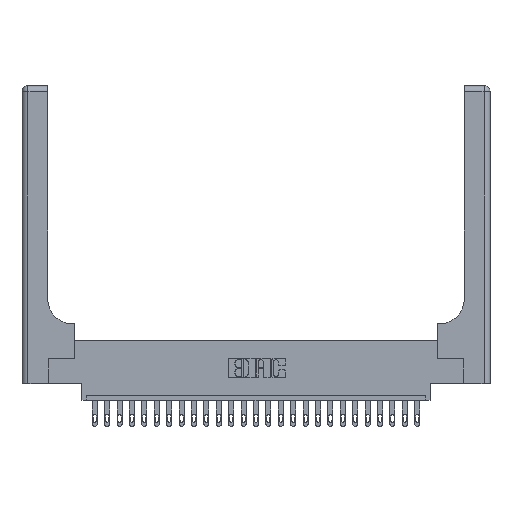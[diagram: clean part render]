
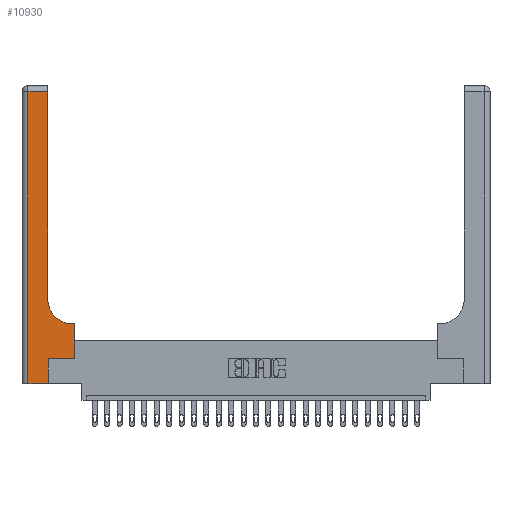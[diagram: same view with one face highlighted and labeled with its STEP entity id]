
A CAD part, top view. The second image highlights one B-rep face of the part: STEP entity #10930.
In plain terms, the highlighted planar face has unit normal (0, 0, 1).
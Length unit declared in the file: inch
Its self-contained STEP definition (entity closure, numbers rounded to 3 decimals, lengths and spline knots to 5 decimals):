
#193 = DIRECTION ( 'NONE',  ( 0., -1., 0. ) ) ;
#1025 = VECTOR ( 'NONE', #5965, 39.37008 ) ;
#1314 = CARTESIAN_POINT ( 'NONE',  ( 0.26, 3., 0.37 ) ) ;
#2083 = VERTEX_POINT ( 'NONE', #12073 ) ;
#2112 = CARTESIAN_POINT ( 'NONE',  ( 0.26, 0.6, 0.37 ) ) ;
#2118 = CARTESIAN_POINT ( 'NONE',  ( 0., 0., 0.37 ) ) ;
#2590 = ORIENTED_EDGE ( 'NONE', *, *, #4494, .T. ) ;
#2878 = CIRCLE ( 'NONE', #19858, 0.25 ) ;
#3769 = DIRECTION ( 'NONE',  ( 0., 0., -1. ) ) ;
#4019 = VERTEX_POINT ( 'NONE', #12612 ) ;
#4285 = CARTESIAN_POINT ( 'NONE',  ( 0.06, 3., 0.37 ) ) ;
#4494 = EDGE_CURVE ( 'NONE', #22353, #8426, #23969, .T. ) ;
#4705 = VERTEX_POINT ( 'NONE', #7761 ) ;
#5190 = LINE ( 'NONE', #10994, #24122 ) ;
#5436 = ORIENTED_EDGE ( 'NONE', *, *, #13300, .T. ) ;
#5561 = EDGE_CURVE ( 'NONE', #14327, #8097, #8085, .T. ) ;
#5607 = CARTESIAN_POINT ( 'NONE',  ( 0.265, 0.25, 0.37 ) ) ;
#5965 = DIRECTION ( 'NONE',  ( 1., 0., 0. ) ) ;
#6201 = CARTESIAN_POINT ( 'NONE',  ( 0.265, 0.25, 0.37 ) ) ;
#7761 = CARTESIAN_POINT ( 'NONE',  ( 0.528, 0.6, 0.37 ) ) ;
#8085 = LINE ( 'NONE', #2118, #1025 ) ;
#8097 = VERTEX_POINT ( 'NONE', #18215 ) ;
#8426 = VERTEX_POINT ( 'NONE', #12751 ) ;
#8872 = ORIENTED_EDGE ( 'NONE', *, *, #14908, .T. ) ;
#9012 = AXIS2_PLACEMENT_3D ( 'NONE', #9348, #3769, #18844 ) ;
#9214 = VECTOR ( 'NONE', #193, 39.37008 ) ;
#9348 = CARTESIAN_POINT ( 'NONE',  ( 0., 3., 0.37 ) ) ;
#10297 = CARTESIAN_POINT ( 'NONE',  ( 0.26, 2.94, 0.37 ) ) ;
#10626 = DIRECTION ( 'NONE',  ( 0., 1., 0. ) ) ;
#10748 = LINE ( 'NONE', #16184, #13868 ) ;
#10930 = ADVANCED_FACE ( 'NONE', ( #11815 ), #19348, .F. ) ;
#10994 = CARTESIAN_POINT ( 'NONE',  ( 0.528, 0.25, 0.37 ) ) ;
#11377 = ORIENTED_EDGE ( 'NONE', *, *, #5561, .T. ) ;
#11395 = DIRECTION ( 'NONE',  ( -1., 0., 0. ) ) ;
#11425 = VECTOR ( 'NONE', #15030, 39.37008 ) ;
#11815 = FACE_OUTER_BOUND ( 'NONE', #22078, .T. ) ;
#12008 = EDGE_CURVE ( 'NONE', #17286, #22353, #12692, .T. ) ;
#12073 = CARTESIAN_POINT ( 'NONE',  ( 0.528, 0.25, 0.37 ) ) ;
#12216 = CARTESIAN_POINT ( 'NONE',  ( 0.51, 0.85, 0.37 ) ) ;
#12612 = CARTESIAN_POINT ( 'NONE',  ( 0.51, 0.6, 0.37 ) ) ;
#12692 = LINE ( 'NONE', #1314, #11425 ) ;
#12751 = CARTESIAN_POINT ( 'NONE',  ( 0.06, 2.94, 0.37 ) ) ;
#13104 = VERTEX_POINT ( 'NONE', #6201 ) ;
#13300 = EDGE_CURVE ( 'NONE', #2083, #4705, #5190, .T. ) ;
#13559 = VECTOR ( 'NONE', #22098, 39.37008 ) ;
#13868 = VECTOR ( 'NONE', #10626, 39.37008 ) ;
#14327 = VERTEX_POINT ( 'NONE', #21493 ) ;
#14553 = CARTESIAN_POINT ( 'NONE',  ( 0., 2.94, 0.37 ) ) ;
#14908 = EDGE_CURVE ( 'NONE', #13104, #2083, #23933, .T. ) ;
#15030 = DIRECTION ( 'NONE',  ( 0., 1., 0. ) ) ;
#15076 = VECTOR ( 'NONE', #22183, 39.37008 ) ;
#15535 = VECTOR ( 'NONE', #11395, 39.37008 ) ;
#15697 = DIRECTION ( 'NONE',  ( 0., 0., -1. ) ) ;
#15782 = LINE ( 'NONE', #4285, #9214 ) ;
#15858 = EDGE_CURVE ( 'NONE', #8426, #14327, #15782, .T. ) ;
#15927 = ORIENTED_EDGE ( 'NONE', *, *, #15858, .T. ) ;
#15940 = CARTESIAN_POINT ( 'NONE',  ( 0.26, 0.85, 0.37 ) ) ;
#16184 = CARTESIAN_POINT ( 'NONE',  ( 0.265, 0., 0.37 ) ) ;
#17286 = VERTEX_POINT ( 'NONE', #15940 ) ;
#17294 = EDGE_CURVE ( 'NONE', #4019, #17286, #2878, .T. ) ;
#17616 = ORIENTED_EDGE ( 'NONE', *, *, #17294, .T. ) ;
#17698 = ORIENTED_EDGE ( 'NONE', *, *, #12008, .T. ) ;
#18037 = ORIENTED_EDGE ( 'NONE', *, *, #22919, .T. ) ;
#18067 = EDGE_CURVE ( 'NONE', #4705, #4019, #20792, .T. ) ;
#18215 = CARTESIAN_POINT ( 'NONE',  ( 0.265, 0., 0.37 ) ) ;
#18314 = ORIENTED_EDGE ( 'NONE', *, *, #18067, .T. ) ;
#18844 = DIRECTION ( 'NONE',  ( -1., 0., 0. ) ) ;
#19348 = PLANE ( 'NONE',  #9012 ) ;
#19858 = AXIS2_PLACEMENT_3D ( 'NONE', #12216, #15697, #21376 ) ;
#20792 = LINE ( 'NONE', #2112, #15535 ) ;
#21376 = DIRECTION ( 'NONE',  ( 1., 0., 0. ) ) ;
#21493 = CARTESIAN_POINT ( 'NONE',  ( 0.06, 0., 0.37 ) ) ;
#22078 = EDGE_LOOP ( 'NONE', ( #17698, #2590, #15927, #11377, #18037, #8872, #5436, #18314, #17616 ) ) ;
#22098 = DIRECTION ( 'NONE',  ( -1., 0., 0. ) ) ;
#22183 = DIRECTION ( 'NONE',  ( 1., 0., 0. ) ) ;
#22252 = DIRECTION ( 'NONE',  ( 0., 1., 0. ) ) ;
#22353 = VERTEX_POINT ( 'NONE', #10297 ) ;
#22919 = EDGE_CURVE ( 'NONE', #8097, #13104, #10748, .T. ) ;
#23933 = LINE ( 'NONE', #5607, #15076 ) ;
#23969 = LINE ( 'NONE', #14553, #13559 ) ;
#24122 = VECTOR ( 'NONE', #22252, 39.37008 ) ;
